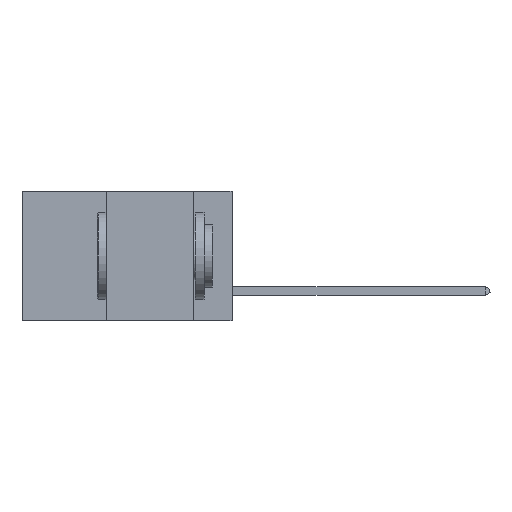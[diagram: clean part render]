
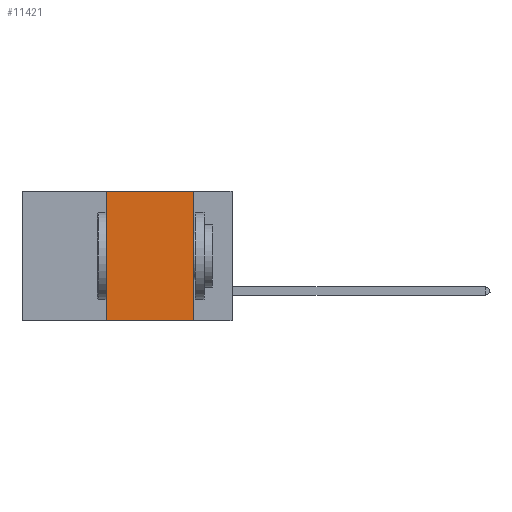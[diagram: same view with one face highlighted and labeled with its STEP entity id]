
A CAD part, left-side view. The second image highlights one B-rep face of the part: STEP entity #11421.
In plain terms, the highlighted planar face has unit normal (-1, 0, 0).
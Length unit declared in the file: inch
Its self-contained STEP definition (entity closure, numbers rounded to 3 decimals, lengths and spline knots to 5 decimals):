
#1017 = EDGE_CURVE ( 'NONE', #1338, #5825, #9804, .T. ) ;
#1082 = LINE ( 'NONE', #2086, #3681 ) ;
#1124 = VERTEX_POINT ( 'NONE', #2154 ) ;
#1315 = ORIENTED_EDGE ( 'NONE', *, *, #10973, .F. ) ;
#1338 = VERTEX_POINT ( 'NONE', #4875 ) ;
#1668 = FACE_OUTER_BOUND ( 'NONE', #9397, .T. ) ;
#1873 = DIRECTION ( 'NONE',  ( 0., -1., 0. ) ) ;
#2086 = CARTESIAN_POINT ( 'NONE',  ( 0., 0.6, -0.37 ) ) ;
#2154 = CARTESIAN_POINT ( 'NONE',  ( 0., 0.11, -0.37 ) ) ;
#2732 = DIRECTION ( 'NONE',  ( 0., 0., 1. ) ) ;
#3681 = VECTOR ( 'NONE', #14827, 39.37008 ) ;
#4069 = ORIENTED_EDGE ( 'NONE', *, *, #6099, .F. ) ;
#4264 = ORIENTED_EDGE ( 'NONE', *, *, #1017, .F. ) ;
#4590 = AXIS2_PLACEMENT_3D ( 'NONE', #7354, #13136, #9669 ) ;
#4875 = CARTESIAN_POINT ( 'NONE',  ( 0., 0.36, -0.37 ) ) ;
#5825 = VERTEX_POINT ( 'NONE', #6300 ) ;
#6099 = EDGE_CURVE ( 'NONE', #14220, #1124, #14585, .T. ) ;
#6300 = CARTESIAN_POINT ( 'NONE',  ( 0., 0.36, 0. ) ) ;
#6537 = CARTESIAN_POINT ( 'NONE',  ( 0., 0.6, 0. ) ) ;
#7354 = CARTESIAN_POINT ( 'NONE',  ( 0., 0.6, 0. ) ) ;
#7534 = VECTOR ( 'NONE', #1873, 39.37008 ) ;
#7858 = CARTESIAN_POINT ( 'NONE',  ( 0., 0.11, 0. ) ) ;
#9397 = EDGE_LOOP ( 'NONE', ( #4069, #1315, #4264, #13866 ) ) ;
#9451 = CARTESIAN_POINT ( 'NONE',  ( 0., 0.11, 0. ) ) ;
#9517 = LINE ( 'NONE', #6537, #7534 ) ;
#9666 = VECTOR ( 'NONE', #13969, 39.37008 ) ;
#9669 = DIRECTION ( 'NONE',  ( 0., 0., -1. ) ) ;
#9690 = CARTESIAN_POINT ( 'NONE',  ( 0., 0.36, 0. ) ) ;
#9804 = LINE ( 'NONE', #9690, #14551 ) ;
#10644 = PLANE ( 'NONE',  #4590 ) ;
#10973 = EDGE_CURVE ( 'NONE', #5825, #14220, #9517, .T. ) ;
#11421 = ADVANCED_FACE ( 'NONE', ( #1668 ), #10644, .F. ) ;
#13136 = DIRECTION ( 'NONE',  ( 1., 0., 0. ) ) ;
#13866 = ORIENTED_EDGE ( 'NONE', *, *, #14155, .T. ) ;
#13969 = DIRECTION ( 'NONE',  ( 0., 0., -1. ) ) ;
#14155 = EDGE_CURVE ( 'NONE', #1338, #1124, #1082, .T. ) ;
#14220 = VERTEX_POINT ( 'NONE', #7858 ) ;
#14551 = VECTOR ( 'NONE', #2732, 39.37008 ) ;
#14585 = LINE ( 'NONE', #9451, #9666 ) ;
#14827 = DIRECTION ( 'NONE',  ( 0., -1., 0. ) ) ;
